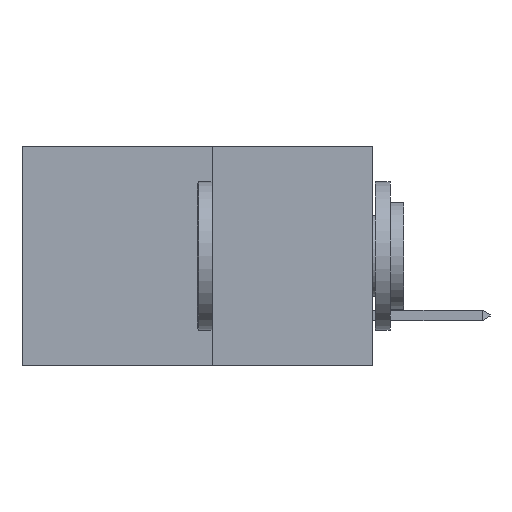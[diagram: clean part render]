
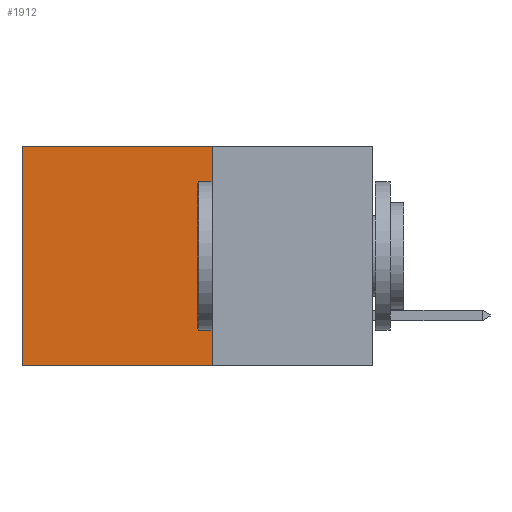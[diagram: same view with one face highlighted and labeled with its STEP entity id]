
A CAD part, left-side view. The second image highlights one B-rep face of the part: STEP entity #1912.
In plain terms, the highlighted planar face has unit normal (-1, 0, 0).
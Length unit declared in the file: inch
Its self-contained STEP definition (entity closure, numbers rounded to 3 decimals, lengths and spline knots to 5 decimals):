
#291 = VERTEX_POINT ( 'NONE', #5606 ) ;
#396 = EDGE_CURVE ( 'NONE', #13200, #291, #6382, .T. ) ;
#1912 = ADVANCED_FACE ( 'NONE', ( #5476 ), #9162, .F. ) ;
#1922 = ORIENTED_EDGE ( 'NONE', *, *, #2283, .F. ) ;
#1997 = ORIENTED_EDGE ( 'NONE', *, *, #6859, .F. ) ;
#2283 = EDGE_CURVE ( 'NONE', #10551, #291, #9652, .T. ) ;
#2723 = DIRECTION ( 'NONE',  ( 0., 1., 0. ) ) ;
#3455 = VECTOR ( 'NONE', #7257, 39.37008 ) ;
#3764 = EDGE_LOOP ( 'NONE', ( #6818, #1922, #1997, #6772 ) ) ;
#3911 = VECTOR ( 'NONE', #9034, 39.37008 ) ;
#4077 = DIRECTION ( 'NONE',  ( 0., 0., -1. ) ) ;
#4502 = DIRECTION ( 'NONE',  ( 1., 0., 0. ) ) ;
#5311 = CARTESIAN_POINT ( 'NONE',  ( 0.277, 0.59, 0. ) ) ;
#5476 = FACE_OUTER_BOUND ( 'NONE', #3764, .T. ) ;
#5555 = CARTESIAN_POINT ( 'NONE',  ( 0.277, 0.27, -0.37 ) ) ;
#5588 = CARTESIAN_POINT ( 'NONE',  ( 0.277, 0.27, -0.37 ) ) ;
#5606 = CARTESIAN_POINT ( 'NONE',  ( 0.277, 0.59, -0.37 ) ) ;
#5706 = DIRECTION ( 'NONE',  ( 0., 0., -1. ) ) ;
#6382 = LINE ( 'NONE', #7429, #3455 ) ;
#6395 = VERTEX_POINT ( 'NONE', #10403 ) ;
#6772 = ORIENTED_EDGE ( 'NONE', *, *, #10155, .T. ) ;
#6818 = ORIENTED_EDGE ( 'NONE', *, *, #396, .T. ) ;
#6859 = EDGE_CURVE ( 'NONE', #6395, #10551, #8710, .T. ) ;
#7102 = CARTESIAN_POINT ( 'NONE',  ( 0.277, 0.27, 0. ) ) ;
#7257 = DIRECTION ( 'NONE',  ( 0., 0., -1. ) ) ;
#7429 = CARTESIAN_POINT ( 'NONE',  ( 0.277, 0.59, -0.37 ) ) ;
#7654 = VECTOR ( 'NONE', #2723, 39.37008 ) ;
#7969 = LINE ( 'NONE', #7102, #7654 ) ;
#8392 = VECTOR ( 'NONE', #5706, 39.37008 ) ;
#8710 = LINE ( 'NONE', #5555, #8392 ) ;
#9034 = DIRECTION ( 'NONE',  ( 0., 1., 0. ) ) ;
#9162 = PLANE ( 'NONE',  #10550 ) ;
#9652 = LINE ( 'NONE', #10873, #3911 ) ;
#10155 = EDGE_CURVE ( 'NONE', #6395, #13200, #7969, .T. ) ;
#10403 = CARTESIAN_POINT ( 'NONE',  ( 0.277, 0.27, 0. ) ) ;
#10550 = AXIS2_PLACEMENT_3D ( 'NONE', #10830, #4502, #4077 ) ;
#10551 = VERTEX_POINT ( 'NONE', #5588 ) ;
#10830 = CARTESIAN_POINT ( 'NONE',  ( 0.277, 0.27, -0.37 ) ) ;
#10873 = CARTESIAN_POINT ( 'NONE',  ( 0.277, 0.27, -0.37 ) ) ;
#13200 = VERTEX_POINT ( 'NONE', #5311 ) ;
